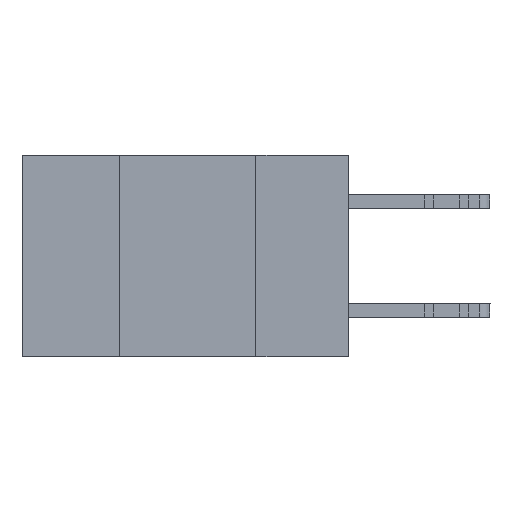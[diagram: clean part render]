
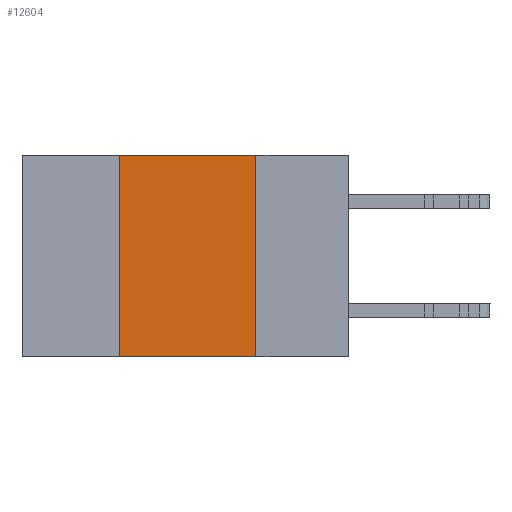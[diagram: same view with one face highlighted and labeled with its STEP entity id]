
A CAD part, left-side view. The second image highlights one B-rep face of the part: STEP entity #12604.
In plain terms, the highlighted planar face has unit normal (-1, 0, 0).
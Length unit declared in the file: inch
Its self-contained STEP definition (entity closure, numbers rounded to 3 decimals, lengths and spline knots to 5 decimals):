
#513 = CARTESIAN_POINT ( 'NONE',  ( 0., 0.42, 0. ) ) ;
#606 = CARTESIAN_POINT ( 'NONE',  ( 0., 0.42, -0.37 ) ) ;
#774 = VECTOR ( 'NONE', #22680, 39.37008 ) ;
#1797 = VERTEX_POINT ( 'NONE', #513 ) ;
#2261 = VECTOR ( 'NONE', #21539, 39.37008 ) ;
#3808 = DIRECTION ( 'NONE',  ( 0., 0., -1. ) ) ;
#4109 = ORIENTED_EDGE ( 'NONE', *, *, #23626, .F. ) ;
#5271 = VERTEX_POINT ( 'NONE', #606 ) ;
#5760 = CARTESIAN_POINT ( 'NONE',  ( 0., 0.17, -0.37 ) ) ;
#6195 = VECTOR ( 'NONE', #8765, 39.37008 ) ;
#7285 = FACE_OUTER_BOUND ( 'NONE', #13620, .T. ) ;
#7378 = CARTESIAN_POINT ( 'NONE',  ( 0., 0.6, 0. ) ) ;
#7570 = LINE ( 'NONE', #5760, #2261 ) ;
#8157 = ORIENTED_EDGE ( 'NONE', *, *, #8192, .T. ) ;
#8192 = EDGE_CURVE ( 'NONE', #5271, #12535, #18662, .T. ) ;
#8765 = DIRECTION ( 'NONE',  ( 0., -1., 0. ) ) ;
#9096 = ORIENTED_EDGE ( 'NONE', *, *, #9174, .F. ) ;
#9174 = EDGE_CURVE ( 'NONE', #1797, #18171, #16190, .T. ) ;
#11464 = LINE ( 'NONE', #20787, #774 ) ;
#11756 = CARTESIAN_POINT ( 'NONE',  ( 0., 0.6, 0. ) ) ;
#12535 = VERTEX_POINT ( 'NONE', #15513 ) ;
#12604 = ADVANCED_FACE ( 'NONE', ( #7285 ), #13779, .F. ) ;
#13236 = EDGE_CURVE ( 'NONE', #18171, #12535, #7570, .T. ) ;
#13620 = EDGE_LOOP ( 'NONE', ( #20226, #9096, #4109, #8157 ) ) ;
#13779 = PLANE ( 'NONE',  #23068 ) ;
#14091 = VECTOR ( 'NONE', #25040, 39.37008 ) ;
#15513 = CARTESIAN_POINT ( 'NONE',  ( 0., 0.17, -0.37 ) ) ;
#15770 = DIRECTION ( 'NONE',  ( 1., 0., 0. ) ) ;
#15955 = CARTESIAN_POINT ( 'NONE',  ( 0., 0.17, 0. ) ) ;
#16190 = LINE ( 'NONE', #7378, #6195 ) ;
#18171 = VERTEX_POINT ( 'NONE', #15955 ) ;
#18662 = LINE ( 'NONE', #25182, #14091 ) ;
#20226 = ORIENTED_EDGE ( 'NONE', *, *, #13236, .F. ) ;
#20787 = CARTESIAN_POINT ( 'NONE',  ( 0., 0.42, -0.37 ) ) ;
#21539 = DIRECTION ( 'NONE',  ( 0., 0., -1. ) ) ;
#22680 = DIRECTION ( 'NONE',  ( 0., 0., 1. ) ) ;
#23068 = AXIS2_PLACEMENT_3D ( 'NONE', #11756, #15770, #3808 ) ;
#23626 = EDGE_CURVE ( 'NONE', #5271, #1797, #11464, .T. ) ;
#25040 = DIRECTION ( 'NONE',  ( 0., -1., 0. ) ) ;
#25182 = CARTESIAN_POINT ( 'NONE',  ( 0., 0.6, -0.37 ) ) ;
